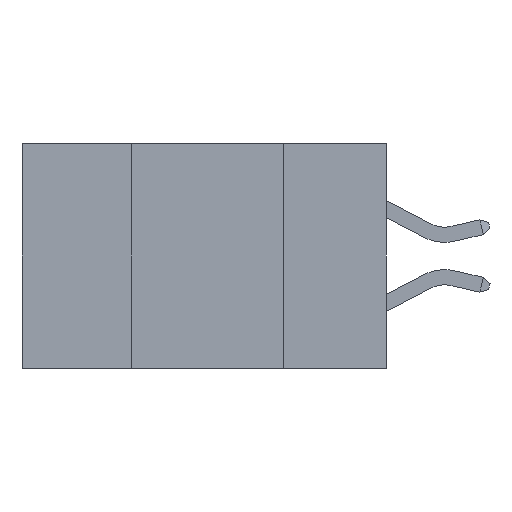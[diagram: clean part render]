
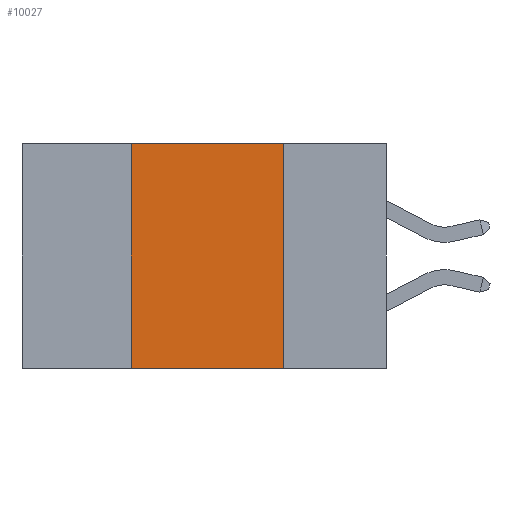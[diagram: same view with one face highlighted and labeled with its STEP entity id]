
A CAD part, left-side view. The second image highlights one B-rep face of the part: STEP entity #10027.
In plain terms, the highlighted planar face has unit normal (-1, 0, 0).
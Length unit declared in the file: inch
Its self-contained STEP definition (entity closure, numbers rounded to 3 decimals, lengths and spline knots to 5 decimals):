
#633 = EDGE_LOOP ( 'NONE', ( #16622, #13071, #1313, #18452 ) ) ;
#984 = DIRECTION ( 'NONE',  ( 1., 0., 0. ) ) ;
#1313 = ORIENTED_EDGE ( 'NONE', *, *, #16764, .F. ) ;
#1352 = CARTESIAN_POINT ( 'NONE',  ( 0., 0.6, -0.37 ) ) ;
#1376 = CARTESIAN_POINT ( 'NONE',  ( 0., 0.6, 0. ) ) ;
#3597 = LINE ( 'NONE', #1352, #19242 ) ;
#3812 = CARTESIAN_POINT ( 'NONE',  ( 0., 0.42, -0.37 ) ) ;
#5646 = VECTOR ( 'NONE', #13653, 39.37008 ) ;
#6040 = CARTESIAN_POINT ( 'NONE',  ( 0., 0.17, 0. ) ) ;
#7158 = DIRECTION ( 'NONE',  ( 0., 0., 1. ) ) ;
#7487 = CARTESIAN_POINT ( 'NONE',  ( 0., 0.42, 0. ) ) ;
#7903 = VECTOR ( 'NONE', #7158, 39.37008 ) ;
#8046 = VECTOR ( 'NONE', #18233, 39.37008 ) ;
#8358 = LINE ( 'NONE', #17747, #7903 ) ;
#8896 = VERTEX_POINT ( 'NONE', #6040 ) ;
#8990 = DIRECTION ( 'NONE',  ( 0., -1., 0. ) ) ;
#9484 = VERTEX_POINT ( 'NONE', #7487 ) ;
#9601 = EDGE_CURVE ( 'NONE', #8896, #13291, #12126, .T. ) ;
#9822 = CARTESIAN_POINT ( 'NONE',  ( 0., 0.17, -0.37 ) ) ;
#10027 = ADVANCED_FACE ( 'NONE', ( #12110 ), #16248, .F. ) ;
#10178 = CARTESIAN_POINT ( 'NONE',  ( 0., 0.6, 0. ) ) ;
#11673 = EDGE_CURVE ( 'NONE', #9484, #8896, #13758, .T. ) ;
#11722 = DIRECTION ( 'NONE',  ( 0., 0., -1. ) ) ;
#12110 = FACE_OUTER_BOUND ( 'NONE', #633, .T. ) ;
#12126 = LINE ( 'NONE', #16781, #8046 ) ;
#13071 = ORIENTED_EDGE ( 'NONE', *, *, #11673, .F. ) ;
#13291 = VERTEX_POINT ( 'NONE', #9822 ) ;
#13308 = VERTEX_POINT ( 'NONE', #3812 ) ;
#13653 = DIRECTION ( 'NONE',  ( 0., -1., 0. ) ) ;
#13758 = LINE ( 'NONE', #1376, #5646 ) ;
#14756 = EDGE_CURVE ( 'NONE', #13308, #13291, #3597, .T. ) ;
#15274 = AXIS2_PLACEMENT_3D ( 'NONE', #10178, #984, #11722 ) ;
#16248 = PLANE ( 'NONE',  #15274 ) ;
#16622 = ORIENTED_EDGE ( 'NONE', *, *, #9601, .F. ) ;
#16764 = EDGE_CURVE ( 'NONE', #13308, #9484, #8358, .T. ) ;
#16781 = CARTESIAN_POINT ( 'NONE',  ( 0., 0.17, -0.37 ) ) ;
#17747 = CARTESIAN_POINT ( 'NONE',  ( 0., 0.42, -0.37 ) ) ;
#18233 = DIRECTION ( 'NONE',  ( 0., 0., -1. ) ) ;
#18452 = ORIENTED_EDGE ( 'NONE', *, *, #14756, .T. ) ;
#19242 = VECTOR ( 'NONE', #8990, 39.37008 ) ;
